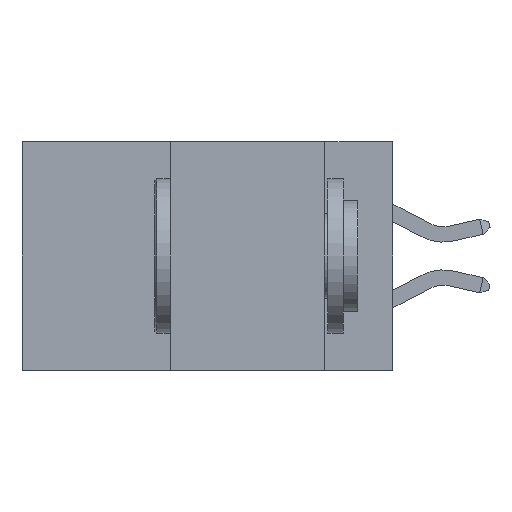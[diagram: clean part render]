
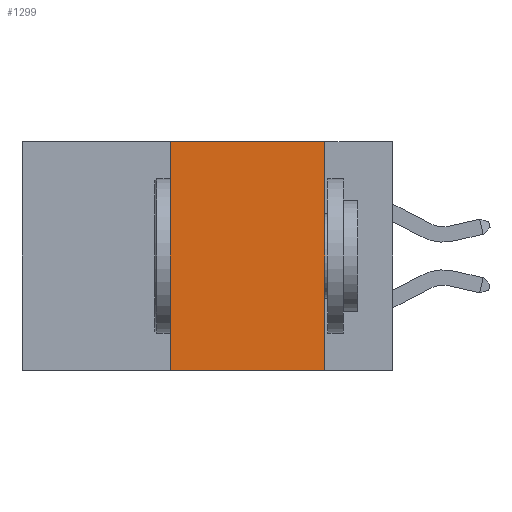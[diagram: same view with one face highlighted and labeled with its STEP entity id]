
A CAD part, left-side view. The second image highlights one B-rep face of the part: STEP entity #1299.
In plain terms, the highlighted planar face has unit normal (-1, 0, 0).
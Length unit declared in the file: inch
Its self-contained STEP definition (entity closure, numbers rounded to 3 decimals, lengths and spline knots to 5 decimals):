
#1299 = ADVANCED_FACE ( 'NONE', ( #1875 ), #3685, .F. ) ;
#1875 = FACE_OUTER_BOUND ( 'NONE', #29339, .T. ) ;
#3345 = LINE ( 'NONE', #13800, #15795 ) ;
#3685 = PLANE ( 'NONE',  #20302 ) ;
#5190 = VECTOR ( 'NONE', #7172, 39.37008 ) ;
#5969 = DIRECTION ( 'NONE',  ( 0., 0., -1. ) ) ;
#7172 = DIRECTION ( 'NONE',  ( 0., -1., 0. ) ) ;
#7589 = VECTOR ( 'NONE', #20506, 39.37008 ) ;
#8178 = DIRECTION ( 'NONE',  ( 0., 0., -1. ) ) ;
#8204 = VERTEX_POINT ( 'NONE', #18221 ) ;
#8209 = CARTESIAN_POINT ( 'NONE',  ( 0., 0.36, 0. ) ) ;
#9443 = ORIENTED_EDGE ( 'NONE', *, *, #23042, .T. ) ;
#10218 = CARTESIAN_POINT ( 'NONE',  ( 0., 0.6, 0. ) ) ;
#10265 = LINE ( 'NONE', #21849, #5190 ) ;
#11459 = DIRECTION ( 'NONE',  ( 1., 0., 0. ) ) ;
#13800 = CARTESIAN_POINT ( 'NONE',  ( 0., 0.6, 0. ) ) ;
#14610 = VECTOR ( 'NONE', #5969, 39.37008 ) ;
#15795 = VECTOR ( 'NONE', #30867, 39.37008 ) ;
#16548 = VERTEX_POINT ( 'NONE', #18753 ) ;
#18221 = CARTESIAN_POINT ( 'NONE',  ( 0., 0.36, 0. ) ) ;
#18753 = CARTESIAN_POINT ( 'NONE',  ( 0., 0.11, 0. ) ) ;
#20302 = AXIS2_PLACEMENT_3D ( 'NONE', #10218, #11459, #8178 ) ;
#20393 = EDGE_CURVE ( 'NONE', #8204, #16548, #3345, .T. ) ;
#20506 = DIRECTION ( 'NONE',  ( 0., 0., 1. ) ) ;
#20653 = CARTESIAN_POINT ( 'NONE',  ( 0., 0.11, 0. ) ) ;
#21373 = LINE ( 'NONE', #8209, #7589 ) ;
#21670 = ORIENTED_EDGE ( 'NONE', *, *, #27975, .F. ) ;
#21849 = CARTESIAN_POINT ( 'NONE',  ( 0., 0.6, -0.37 ) ) ;
#23042 = EDGE_CURVE ( 'NONE', #24518, #28645, #10265, .T. ) ;
#24518 = VERTEX_POINT ( 'NONE', #29726 ) ;
#25451 = CARTESIAN_POINT ( 'NONE',  ( 0., 0.11, -0.37 ) ) ;
#26807 = LINE ( 'NONE', #20653, #14610 ) ;
#27349 = EDGE_CURVE ( 'NONE', #16548, #28645, #26807, .T. ) ;
#27436 = ORIENTED_EDGE ( 'NONE', *, *, #27349, .F. ) ;
#27975 = EDGE_CURVE ( 'NONE', #24518, #8204, #21373, .T. ) ;
#28645 = VERTEX_POINT ( 'NONE', #25451 ) ;
#29339 = EDGE_LOOP ( 'NONE', ( #27436, #29356, #21670, #9443 ) ) ;
#29356 = ORIENTED_EDGE ( 'NONE', *, *, #20393, .F. ) ;
#29726 = CARTESIAN_POINT ( 'NONE',  ( 0., 0.36, -0.37 ) ) ;
#30867 = DIRECTION ( 'NONE',  ( 0., -1., 0. ) ) ;
